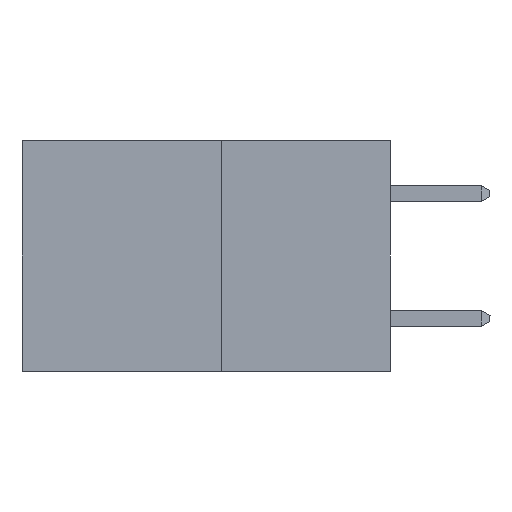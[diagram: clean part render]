
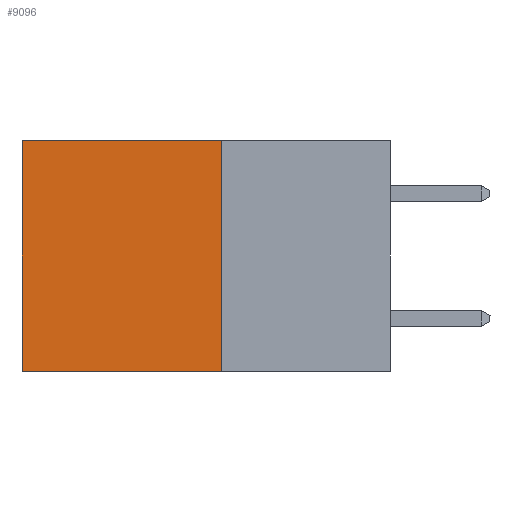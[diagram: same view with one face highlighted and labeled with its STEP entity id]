
A CAD part, left-side view. The second image highlights one B-rep face of the part: STEP entity #9096.
In plain terms, the highlighted planar face has unit normal (-1, 0, 0).
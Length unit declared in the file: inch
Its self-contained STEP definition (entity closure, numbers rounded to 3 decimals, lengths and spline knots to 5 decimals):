
#22 = DIRECTION ( 'NONE',  ( 0., 0., -1. ) ) ;
#225 = VERTEX_POINT ( 'NONE', #5227 ) ;
#292 = EDGE_CURVE ( 'NONE', #225, #9128, #2660, .T. ) ;
#858 = EDGE_CURVE ( 'NONE', #9128, #5182, #6694, .T. ) ;
#939 = VECTOR ( 'NONE', #8988, 39.37008 ) ;
#2176 = PLANE ( 'NONE',  #8983 ) ;
#2215 = CARTESIAN_POINT ( 'NONE',  ( 0.277, 0.27, -0.37 ) ) ;
#2216 = EDGE_LOOP ( 'NONE', ( #6444, #7511, #2614, #3098 ) ) ;
#2614 = ORIENTED_EDGE ( 'NONE', *, *, #292, .F. ) ;
#2637 = EDGE_CURVE ( 'NONE', #6489, #5182, #3175, .T. ) ;
#2660 = LINE ( 'NONE', #7286, #8132 ) ;
#3098 = ORIENTED_EDGE ( 'NONE', *, *, #4938, .T. ) ;
#3175 = LINE ( 'NONE', #4112, #5406 ) ;
#3430 = FACE_OUTER_BOUND ( 'NONE', #2216, .T. ) ;
#3601 = CARTESIAN_POINT ( 'NONE',  ( 0.277, 0.59, -0.37 ) ) ;
#3732 = DIRECTION ( 'NONE',  ( 0., 0., -1. ) ) ;
#3916 = DIRECTION ( 'NONE',  ( 0., 1., 0. ) ) ;
#4112 = CARTESIAN_POINT ( 'NONE',  ( 0.277, 0.59, -0.37 ) ) ;
#4240 = DIRECTION ( 'NONE',  ( 0., 0., -1. ) ) ;
#4938 = EDGE_CURVE ( 'NONE', #225, #6489, #7204, .T. ) ;
#5182 = VERTEX_POINT ( 'NONE', #3601 ) ;
#5227 = CARTESIAN_POINT ( 'NONE',  ( 0.277, 0.27, 0. ) ) ;
#5406 = VECTOR ( 'NONE', #4240, 39.37008 ) ;
#6444 = ORIENTED_EDGE ( 'NONE', *, *, #2637, .T. ) ;
#6489 = VERTEX_POINT ( 'NONE', #7196 ) ;
#6673 = CARTESIAN_POINT ( 'NONE',  ( 0.277, 0.27, -0.37 ) ) ;
#6694 = LINE ( 'NONE', #6673, #939 ) ;
#6747 = VECTOR ( 'NONE', #3916, 39.37008 ) ;
#6844 = CARTESIAN_POINT ( 'NONE',  ( 0.277, 0.27, 0. ) ) ;
#7196 = CARTESIAN_POINT ( 'NONE',  ( 0.277, 0.59, 0. ) ) ;
#7204 = LINE ( 'NONE', #6844, #6747 ) ;
#7286 = CARTESIAN_POINT ( 'NONE',  ( 0.277, 0.27, -0.37 ) ) ;
#7411 = CARTESIAN_POINT ( 'NONE',  ( 0.277, 0.27, -0.37 ) ) ;
#7511 = ORIENTED_EDGE ( 'NONE', *, *, #858, .F. ) ;
#8132 = VECTOR ( 'NONE', #22, 39.37008 ) ;
#8143 = DIRECTION ( 'NONE',  ( 1., 0., 0. ) ) ;
#8983 = AXIS2_PLACEMENT_3D ( 'NONE', #7411, #8143, #3732 ) ;
#8988 = DIRECTION ( 'NONE',  ( 0., 1., 0. ) ) ;
#9096 = ADVANCED_FACE ( 'NONE', ( #3430 ), #2176, .F. ) ;
#9128 = VERTEX_POINT ( 'NONE', #2215 ) ;
